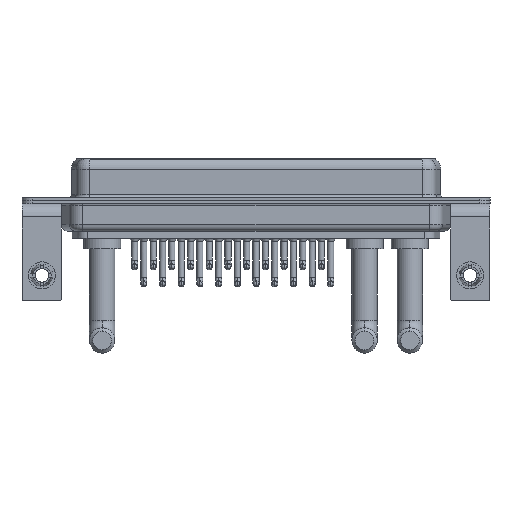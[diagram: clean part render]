
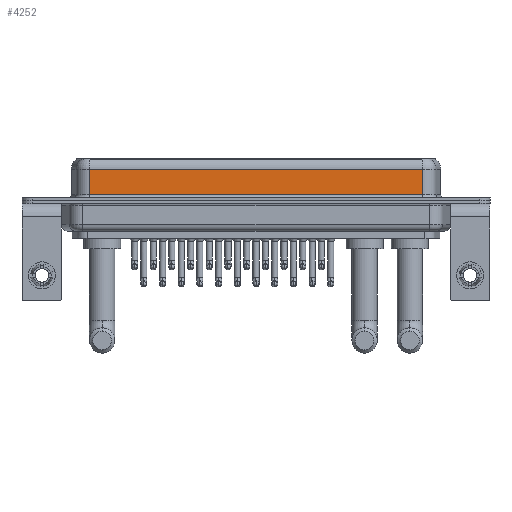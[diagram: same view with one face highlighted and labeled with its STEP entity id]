
A CAD part, front view. The second image highlights one B-rep face of the part: STEP entity #4252.
In plain terms, the highlighted planar face has unit normal (0, -1, 0).
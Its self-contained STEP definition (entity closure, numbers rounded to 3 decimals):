
#1513 = ORIENTED_EDGE ( 'NONE', *, *, #22190, .T. ) ;
#2389 = EDGE_LOOP ( 'NONE', ( #10629, #1513, #14399, #8952 ) ) ;
#2527 = EDGE_CURVE ( 'NONE', #21571, #18637, #21433, .T. ) ;
#2731 = EDGE_CURVE ( 'NONE', #18637, #26137, #15259, .T. ) ;
#3260 = CARTESIAN_POINT ( 'NONE',  ( 7.038, -3.95, 6.4 ) ) ;
#4218 = LINE ( 'NONE', #16288, #7407 ) ;
#4252 = ADVANCED_FACE ( 'NONE', ( #23655 ), #11456, .F. ) ;
#4845 = CARTESIAN_POINT ( 'NONE',  ( 56.462, -3.95, 4.65 ) ) ;
#6112 = VECTOR ( 'NONE', #21397, 1000. ) ;
#7063 = CARTESIAN_POINT ( 'NONE',  ( 56.462, -3.95, 0.9 ) ) ;
#7407 = VECTOR ( 'NONE', #20409, 1000. ) ;
#7748 = CARTESIAN_POINT ( 'NONE',  ( 56.462, -3.95, 4.65 ) ) ;
#8248 = CARTESIAN_POINT ( 'NONE',  ( 56.462, -3.95, 0.9 ) ) ;
#8952 = ORIENTED_EDGE ( 'NONE', *, *, #2731, .T. ) ;
#9197 = VECTOR ( 'NONE', #11355, 1000. ) ;
#9851 = VECTOR ( 'NONE', #11297, 1000. ) ;
#10476 = CARTESIAN_POINT ( 'NONE',  ( 7.038, -3.95, 0.9 ) ) ;
#10629 = ORIENTED_EDGE ( 'NONE', *, *, #24487, .F. ) ;
#11201 = CARTESIAN_POINT ( 'NONE',  ( 56.462, -3.95, 6.4 ) ) ;
#11297 = DIRECTION ( 'NONE',  ( 1., 0., 0. ) ) ;
#11355 = DIRECTION ( 'NONE',  ( 0., 0., -1. ) ) ;
#11456 = PLANE ( 'NONE',  #19454 ) ;
#11714 = VERTEX_POINT ( 'NONE', #4845 ) ;
#12784 = CARTESIAN_POINT ( 'NONE',  ( 7.038, -3.95, 4.65 ) ) ;
#14399 = ORIENTED_EDGE ( 'NONE', *, *, #2527, .T. ) ;
#15259 = LINE ( 'NONE', #7063, #9851 ) ;
#16288 = CARTESIAN_POINT ( 'NONE',  ( 56.462, -3.95, 6.4 ) ) ;
#17404 = LINE ( 'NONE', #7748, #6112 ) ;
#17681 = DIRECTION ( 'NONE',  ( 0., 1., 0. ) ) ;
#18637 = VERTEX_POINT ( 'NONE', #10476 ) ;
#19454 = AXIS2_PLACEMENT_3D ( 'NONE', #11201, #17681, #25635 ) ;
#20409 = DIRECTION ( 'NONE',  ( 0., 0., -1. ) ) ;
#21397 = DIRECTION ( 'NONE',  ( -1., 0., 0. ) ) ;
#21433 = LINE ( 'NONE', #3260, #9197 ) ;
#21571 = VERTEX_POINT ( 'NONE', #12784 ) ;
#22190 = EDGE_CURVE ( 'NONE', #11714, #21571, #17404, .T. ) ;
#23655 = FACE_OUTER_BOUND ( 'NONE', #2389, .T. ) ;
#24487 = EDGE_CURVE ( 'NONE', #11714, #26137, #4218, .T. ) ;
#25635 = DIRECTION ( 'NONE',  ( 0., 0., 1. ) ) ;
#26137 = VERTEX_POINT ( 'NONE', #8248 ) ;
